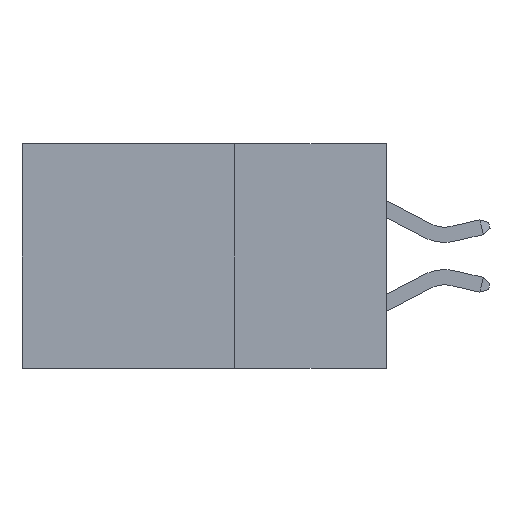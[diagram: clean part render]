
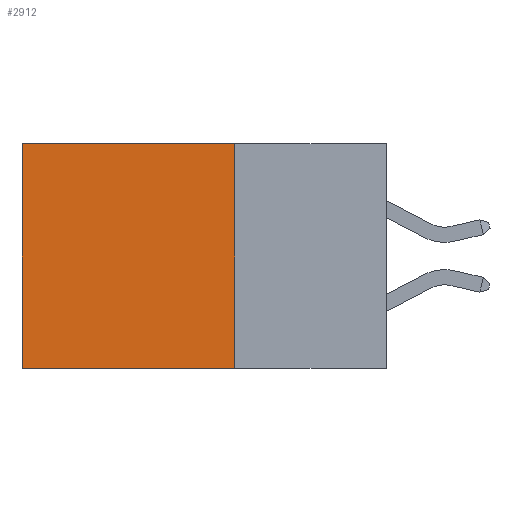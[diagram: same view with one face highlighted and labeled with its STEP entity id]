
A CAD part, left-side view. The second image highlights one B-rep face of the part: STEP entity #2912.
In plain terms, the highlighted planar face has unit normal (-1, 0, 0).
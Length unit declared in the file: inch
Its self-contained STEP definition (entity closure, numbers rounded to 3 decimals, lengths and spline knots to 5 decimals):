
#15 = CARTESIAN_POINT ( 'NONE',  ( 0.2615, 0.25, 0. ) ) ;
#837 = LINE ( 'NONE', #9564, #14455 ) ;
#920 = DIRECTION ( 'NONE',  ( 0., 0., -1. ) ) ;
#1186 = EDGE_CURVE ( 'NONE', #4091, #5488, #4287, .T. ) ;
#1803 = VECTOR ( 'NONE', #15558, 39.37008 ) ;
#2541 = VERTEX_POINT ( 'NONE', #14037 ) ;
#2613 = ORIENTED_EDGE ( 'NONE', *, *, #2698, .T. ) ;
#2698 = EDGE_CURVE ( 'NONE', #5488, #13909, #837, .T. ) ;
#2718 = EDGE_CURVE ( 'NONE', #2541, #13909, #4802, .T. ) ;
#2813 = EDGE_LOOP ( 'NONE', ( #2613, #3776, #7719, #6369 ) ) ;
#2912 = ADVANCED_FACE ( 'NONE', ( #4843 ), #7272, .F. ) ;
#3081 = DIRECTION ( 'NONE',  ( 0., 1., 0. ) ) ;
#3776 = ORIENTED_EDGE ( 'NONE', *, *, #2718, .F. ) ;
#4091 = VERTEX_POINT ( 'NONE', #15 ) ;
#4287 = LINE ( 'NONE', #14165, #7454 ) ;
#4518 = LINE ( 'NONE', #4668, #4958 ) ;
#4668 = CARTESIAN_POINT ( 'NONE',  ( 0.2615, 0.25, -0.37 ) ) ;
#4802 = LINE ( 'NONE', #9942, #1803 ) ;
#4843 = FACE_OUTER_BOUND ( 'NONE', #2813, .T. ) ;
#4958 = VECTOR ( 'NONE', #7015, 39.37008 ) ;
#5488 = VERTEX_POINT ( 'NONE', #10435 ) ;
#6369 = ORIENTED_EDGE ( 'NONE', *, *, #1186, .T. ) ;
#7015 = DIRECTION ( 'NONE',  ( 0., 0., -1. ) ) ;
#7272 = PLANE ( 'NONE',  #8085 ) ;
#7454 = VECTOR ( 'NONE', #3081, 39.37008 ) ;
#7719 = ORIENTED_EDGE ( 'NONE', *, *, #13069, .F. ) ;
#8085 = AXIS2_PLACEMENT_3D ( 'NONE', #12368, #8388, #8620 ) ;
#8388 = DIRECTION ( 'NONE',  ( 1., 0., 0. ) ) ;
#8415 = CARTESIAN_POINT ( 'NONE',  ( 0.2615, 0.6, -0.37 ) ) ;
#8620 = DIRECTION ( 'NONE',  ( 0., 0., -1. ) ) ;
#9564 = CARTESIAN_POINT ( 'NONE',  ( 0.2615, 0.6, -0.37 ) ) ;
#9942 = CARTESIAN_POINT ( 'NONE',  ( 0.2615, 0.25, -0.37 ) ) ;
#10435 = CARTESIAN_POINT ( 'NONE',  ( 0.2615, 0.6, 0. ) ) ;
#12368 = CARTESIAN_POINT ( 'NONE',  ( 0.2615, 0.25, -0.37 ) ) ;
#13069 = EDGE_CURVE ( 'NONE', #4091, #2541, #4518, .T. ) ;
#13909 = VERTEX_POINT ( 'NONE', #8415 ) ;
#14037 = CARTESIAN_POINT ( 'NONE',  ( 0.2615, 0.25, -0.37 ) ) ;
#14165 = CARTESIAN_POINT ( 'NONE',  ( 0.2615, 0.25, 0. ) ) ;
#14455 = VECTOR ( 'NONE', #920, 39.37008 ) ;
#15558 = DIRECTION ( 'NONE',  ( 0., 1., 0. ) ) ;
